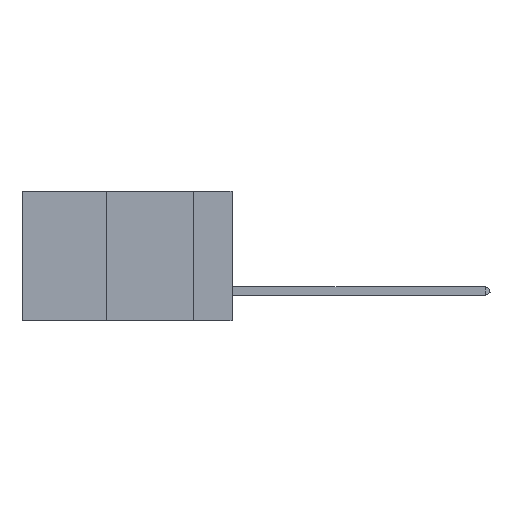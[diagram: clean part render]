
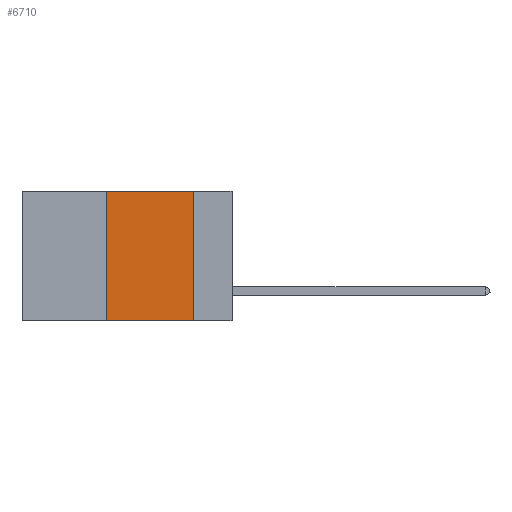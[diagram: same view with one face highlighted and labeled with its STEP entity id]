
A CAD part, left-side view. The second image highlights one B-rep face of the part: STEP entity #6710.
In plain terms, the highlighted planar face has unit normal (-1, 0, 0).
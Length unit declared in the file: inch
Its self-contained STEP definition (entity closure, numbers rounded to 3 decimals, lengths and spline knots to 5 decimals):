
#19 = ORIENTED_EDGE ( 'NONE', *, *, #15841, .F. ) ;
#266 = VERTEX_POINT ( 'NONE', #8249 ) ;
#520 = CARTESIAN_POINT ( 'NONE',  ( 0., 0.36, -0.37 ) ) ;
#2350 = CARTESIAN_POINT ( 'NONE',  ( 0., 0.6, 0. ) ) ;
#2382 = PLANE ( 'NONE',  #5076 ) ;
#3422 = DIRECTION ( 'NONE',  ( 0., 0., -1. ) ) ;
#3826 = CARTESIAN_POINT ( 'NONE',  ( 0., 0.36, 0. ) ) ;
#4232 = CARTESIAN_POINT ( 'NONE',  ( 0., 0.6, 0. ) ) ;
#5076 = AXIS2_PLACEMENT_3D ( 'NONE', #4232, #21290, #11835 ) ;
#6388 = VERTEX_POINT ( 'NONE', #520 ) ;
#6710 = ADVANCED_FACE ( 'NONE', ( #15434 ), #2382, .F. ) ;
#6733 = VECTOR ( 'NONE', #17533, 39.37008 ) ;
#7906 = DIRECTION ( 'NONE',  ( 0., -1., 0. ) ) ;
#8202 = VECTOR ( 'NONE', #3422, 39.37008 ) ;
#8249 = CARTESIAN_POINT ( 'NONE',  ( 0., 0.36, 0. ) ) ;
#8347 = EDGE_CURVE ( 'NONE', #266, #14938, #19382, .T. ) ;
#9553 = DIRECTION ( 'NONE',  ( 0., 0., 1. ) ) ;
#9805 = LINE ( 'NONE', #3826, #19526 ) ;
#9824 = CARTESIAN_POINT ( 'NONE',  ( 0., 0.11, -0.37 ) ) ;
#10216 = ORIENTED_EDGE ( 'NONE', *, *, #21861, .F. ) ;
#11101 = ORIENTED_EDGE ( 'NONE', *, *, #8347, .F. ) ;
#11835 = DIRECTION ( 'NONE',  ( 0., 0., -1. ) ) ;
#12025 = CARTESIAN_POINT ( 'NONE',  ( 0., 0.6, -0.37 ) ) ;
#14495 = CARTESIAN_POINT ( 'NONE',  ( 0., 0.11, 0. ) ) ;
#14938 = VERTEX_POINT ( 'NONE', #14495 ) ;
#15434 = FACE_OUTER_BOUND ( 'NONE', #18050, .T. ) ;
#15841 = EDGE_CURVE ( 'NONE', #6388, #266, #9805, .T. ) ;
#15856 = LINE ( 'NONE', #12025, #23017 ) ;
#16921 = EDGE_CURVE ( 'NONE', #6388, #24223, #15856, .T. ) ;
#17533 = DIRECTION ( 'NONE',  ( 0., -1., 0. ) ) ;
#18050 = EDGE_LOOP ( 'NONE', ( #10216, #11101, #19, #23360 ) ) ;
#19382 = LINE ( 'NONE', #2350, #6733 ) ;
#19526 = VECTOR ( 'NONE', #9553, 39.37008 ) ;
#20583 = LINE ( 'NONE', #22193, #8202 ) ;
#21290 = DIRECTION ( 'NONE',  ( 1., 0., 0. ) ) ;
#21861 = EDGE_CURVE ( 'NONE', #14938, #24223, #20583, .T. ) ;
#22193 = CARTESIAN_POINT ( 'NONE',  ( 0., 0.11, 0. ) ) ;
#23017 = VECTOR ( 'NONE', #7906, 39.37008 ) ;
#23360 = ORIENTED_EDGE ( 'NONE', *, *, #16921, .T. ) ;
#24223 = VERTEX_POINT ( 'NONE', #9824 ) ;
